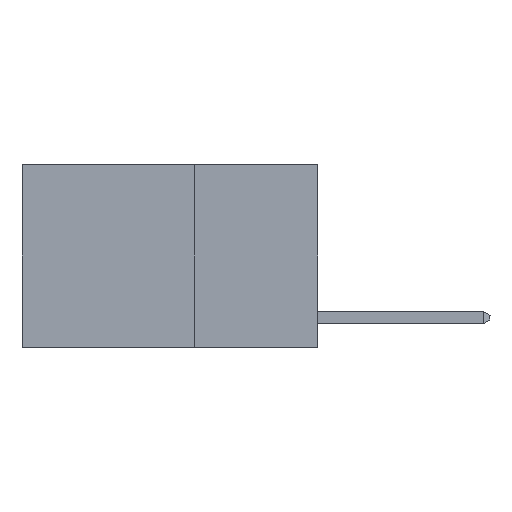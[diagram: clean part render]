
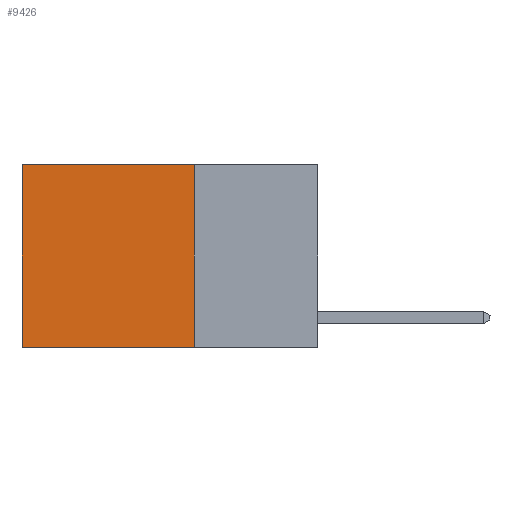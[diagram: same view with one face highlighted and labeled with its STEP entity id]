
A CAD part, left-side view. The second image highlights one B-rep face of the part: STEP entity #9426.
In plain terms, the highlighted planar face has unit normal (-1, 0, 0).
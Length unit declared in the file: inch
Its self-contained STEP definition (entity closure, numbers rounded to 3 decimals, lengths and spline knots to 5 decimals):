
#9 = ORIENTED_EDGE ( 'NONE', *, *, #12520, .T. ) ;
#1438 = ORIENTED_EDGE ( 'NONE', *, *, #21522, .F. ) ;
#2618 = ORIENTED_EDGE ( 'NONE', *, *, #6860, .F. ) ;
#2804 = LINE ( 'NONE', #8048, #7689 ) ;
#3253 = CARTESIAN_POINT ( 'NONE',  ( 0.2625, 0.6, 0. ) ) ;
#3334 = DIRECTION ( 'NONE',  ( 0., 0., -1. ) ) ;
#3563 = LINE ( 'NONE', #3253, #21330 ) ;
#5409 = ORIENTED_EDGE ( 'NONE', *, *, #16392, .T. ) ;
#5576 = VERTEX_POINT ( 'NONE', #8720 ) ;
#6860 = EDGE_CURVE ( 'NONE', #12982, #18174, #2804, .T. ) ;
#7689 = VECTOR ( 'NONE', #9841, 39.37008 ) ;
#8000 = FACE_OUTER_BOUND ( 'NONE', #12283, .T. ) ;
#8048 = CARTESIAN_POINT ( 'NONE',  ( 0.2625, 0.25, -0.37 ) ) ;
#8106 = DIRECTION ( 'NONE',  ( 0., 1., 0. ) ) ;
#8720 = CARTESIAN_POINT ( 'NONE',  ( 0.2625, 0.25, 0. ) ) ;
#8912 = LINE ( 'NONE', #19100, #22354 ) ;
#9325 = VECTOR ( 'NONE', #8106, 39.37008 ) ;
#9426 = ADVANCED_FACE ( 'NONE', ( #8000 ), #22004, .F. ) ;
#9841 = DIRECTION ( 'NONE',  ( 0., 1., 0. ) ) ;
#10136 = DIRECTION ( 'NONE',  ( 1., 0., 0. ) ) ;
#11545 = AXIS2_PLACEMENT_3D ( 'NONE', #20645, #10136, #22392 ) ;
#12283 = EDGE_LOOP ( 'NONE', ( #9, #2618, #1438, #5409 ) ) ;
#12520 = EDGE_CURVE ( 'NONE', #19183, #18174, #3563, .T. ) ;
#12982 = VERTEX_POINT ( 'NONE', #19250 ) ;
#13490 = LINE ( 'NONE', #20414, #9325 ) ;
#14039 = CARTESIAN_POINT ( 'NONE',  ( 0.2625, 0.6, 0. ) ) ;
#14786 = CARTESIAN_POINT ( 'NONE',  ( 0.2625, 0.6, -0.37 ) ) ;
#16392 = EDGE_CURVE ( 'NONE', #5576, #19183, #13490, .T. ) ;
#18174 = VERTEX_POINT ( 'NONE', #14786 ) ;
#19100 = CARTESIAN_POINT ( 'NONE',  ( 0.2625, 0.25, 0. ) ) ;
#19183 = VERTEX_POINT ( 'NONE', #14039 ) ;
#19250 = CARTESIAN_POINT ( 'NONE',  ( 0.2625, 0.25, -0.37 ) ) ;
#20414 = CARTESIAN_POINT ( 'NONE',  ( 0.2625, 0.25, 0. ) ) ;
#20645 = CARTESIAN_POINT ( 'NONE',  ( 0.2625, 0.25, 0. ) ) ;
#20835 = DIRECTION ( 'NONE',  ( 0., 0., -1. ) ) ;
#21330 = VECTOR ( 'NONE', #3334, 39.37008 ) ;
#21522 = EDGE_CURVE ( 'NONE', #5576, #12982, #8912, .T. ) ;
#22004 = PLANE ( 'NONE',  #11545 ) ;
#22354 = VECTOR ( 'NONE', #20835, 39.37008 ) ;
#22392 = DIRECTION ( 'NONE',  ( 0., 0., -1. ) ) ;
